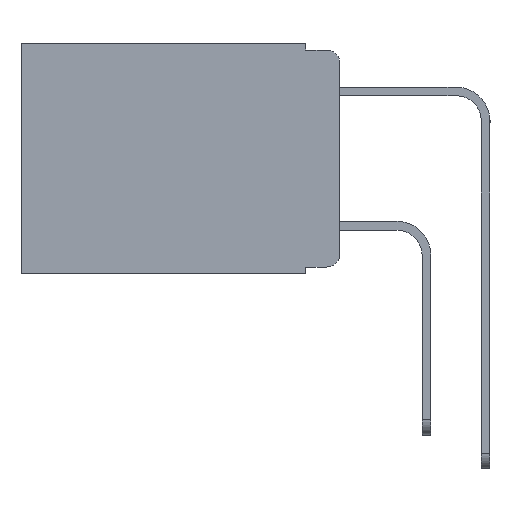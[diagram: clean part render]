
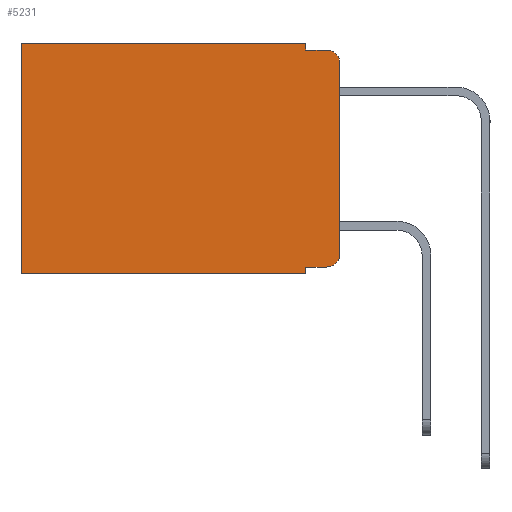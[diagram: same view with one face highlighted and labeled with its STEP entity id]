
A CAD part, left-side view. The second image highlights one B-rep face of the part: STEP entity #5231.
In plain terms, the highlighted planar face has unit normal (-1, 0, 0).
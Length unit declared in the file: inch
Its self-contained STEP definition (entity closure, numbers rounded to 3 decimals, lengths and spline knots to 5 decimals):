
#2 = CARTESIAN_POINT ( 'NONE',  ( 0.298, 0.051, -0.343 ) ) ;
#319 = VERTEX_POINT ( 'NONE', #9623 ) ;
#1503 = CARTESIAN_POINT ( 'NONE',  ( 0.298, 0., -0.343 ) ) ;
#2318 = VERTEX_POINT ( 'NONE', #15195 ) ;
#2337 = ORIENTED_EDGE ( 'NONE', *, *, #12186, .F. ) ;
#2432 = VERTEX_POINT ( 'NONE', #8522 ) ;
#2642 = CARTESIAN_POINT ( 'NONE',  ( 0.298, 0.051, -0.333 ) ) ;
#3061 = VECTOR ( 'NONE', #10099, 39.37008 ) ;
#3215 = CIRCLE ( 'NONE', #21609, 0.02 ) ;
#3262 = ORIENTED_EDGE ( 'NONE', *, *, #10508, .F. ) ;
#3624 = EDGE_CURVE ( 'NONE', #319, #16542, #11801, .T. ) ;
#3670 = DIRECTION ( 'NONE',  ( 1., 0., 0. ) ) ;
#3845 = EDGE_LOOP ( 'NONE', ( #17991, #7827, #21614, #2337, #16322, #11525, #3848, #3262, #21906, #20778 ) ) ;
#3848 = ORIENTED_EDGE ( 'NONE', *, *, #21230, .F. ) ;
#3927 = CARTESIAN_POINT ( 'NONE',  ( 0.298, 0.473, 0. ) ) ;
#3942 = EDGE_CURVE ( 'NONE', #23337, #8528, #10351, .T. ) ;
#4706 = VECTOR ( 'NONE', #10716, 39.37008 ) ;
#4889 = CARTESIAN_POINT ( 'NONE',  ( 0.298, 0.051, -0.01 ) ) ;
#5173 = EDGE_CURVE ( 'NONE', #8528, #9695, #3215, .T. ) ;
#5231 = ADVANCED_FACE ( 'NONE', ( #21304 ), #14564, .F. ) ;
#5513 = VECTOR ( 'NONE', #11139, 39.37008 ) ;
#5578 = DIRECTION ( 'NONE',  ( 0., -1., 0. ) ) ;
#5668 = VECTOR ( 'NONE', #12463, 39.37008 ) ;
#6241 = LINE ( 'NONE', #17768, #5668 ) ;
#6376 = VECTOR ( 'NONE', #5578, 39.37008 ) ;
#6674 = DIRECTION ( 'NONE',  ( 0., 0., -1. ) ) ;
#6680 = AXIS2_PLACEMENT_3D ( 'NONE', #23438, #3670, #16369 ) ;
#7228 = CARTESIAN_POINT ( 'NONE',  ( 0.298, 0.02, -0.01 ) ) ;
#7505 = VECTOR ( 'NONE', #14910, 39.37008 ) ;
#7630 = DIRECTION ( 'NONE',  ( 0., 0., -1. ) ) ;
#7827 = ORIENTED_EDGE ( 'NONE', *, *, #22779, .T. ) ;
#8060 = LINE ( 'NONE', #13087, #7505 ) ;
#8366 = EDGE_CURVE ( 'NONE', #15752, #9695, #8524, .T. ) ;
#8522 = CARTESIAN_POINT ( 'NONE',  ( 0.298, 0.051, 0. ) ) ;
#8524 = LINE ( 'NONE', #11943, #3061 ) ;
#8528 = VERTEX_POINT ( 'NONE', #17709 ) ;
#8738 = DIRECTION ( 'NONE',  ( -1., 0., 0. ) ) ;
#9536 = LINE ( 'NONE', #18415, #15468 ) ;
#9623 = CARTESIAN_POINT ( 'NONE',  ( 0.298, 0.051, -0.01 ) ) ;
#9695 = VERTEX_POINT ( 'NONE', #16052 ) ;
#10099 = DIRECTION ( 'NONE',  ( 0., 0., -1. ) ) ;
#10351 = LINE ( 'NONE', #2642, #5513 ) ;
#10508 = EDGE_CURVE ( 'NONE', #23337, #15420, #9536, .T. ) ;
#10716 = DIRECTION ( 'NONE',  ( 0., 1., 0. ) ) ;
#10855 = CARTESIAN_POINT ( 'NONE',  ( 0.298, 0.02, -0.313 ) ) ;
#10963 = EDGE_CURVE ( 'NONE', #11187, #2318, #6241, .T. ) ;
#11139 = DIRECTION ( 'NONE',  ( 0., -1., 0. ) ) ;
#11187 = VERTEX_POINT ( 'NONE', #3927 ) ;
#11525 = ORIENTED_EDGE ( 'NONE', *, *, #10963, .T. ) ;
#11801 = LINE ( 'NONE', #4889, #6376 ) ;
#11943 = CARTESIAN_POINT ( 'NONE',  ( 0.298, 0., 0. ) ) ;
#12186 = EDGE_CURVE ( 'NONE', #2432, #319, #22229, .T. ) ;
#12463 = DIRECTION ( 'NONE',  ( 0., 0., -1. ) ) ;
#12674 = DIRECTION ( 'NONE',  ( 0., 0., -1. ) ) ;
#13087 = CARTESIAN_POINT ( 'NONE',  ( 0.298, 0., 0. ) ) ;
#14564 = PLANE ( 'NONE',  #6680 ) ;
#14567 = AXIS2_PLACEMENT_3D ( 'NONE', #19501, #8738, #21286 ) ;
#14910 = DIRECTION ( 'NONE',  ( 0., 1., 0. ) ) ;
#15195 = CARTESIAN_POINT ( 'NONE',  ( 0.298, 0.473, -0.343 ) ) ;
#15420 = VERTEX_POINT ( 'NONE', #2 ) ;
#15468 = VECTOR ( 'NONE', #7630, 39.37008 ) ;
#15687 = CARTESIAN_POINT ( 'NONE',  ( 0.298, 0., -0.03 ) ) ;
#15752 = VERTEX_POINT ( 'NONE', #15687 ) ;
#16052 = CARTESIAN_POINT ( 'NONE',  ( 0.298, 0., -0.313 ) ) ;
#16322 = ORIENTED_EDGE ( 'NONE', *, *, #22444, .T. ) ;
#16369 = DIRECTION ( 'NONE',  ( 0., 0., -1. ) ) ;
#16542 = VERTEX_POINT ( 'NONE', #7228 ) ;
#17500 = CARTESIAN_POINT ( 'NONE',  ( 0.298, 0.051, 0. ) ) ;
#17709 = CARTESIAN_POINT ( 'NONE',  ( 0.298, 0.02, -0.333 ) ) ;
#17768 = CARTESIAN_POINT ( 'NONE',  ( 0.298, 0.473, 0. ) ) ;
#17991 = ORIENTED_EDGE ( 'NONE', *, *, #8366, .F. ) ;
#18415 = CARTESIAN_POINT ( 'NONE',  ( 0.298, 0.051, 0. ) ) ;
#19098 = LINE ( 'NONE', #1503, #4706 ) ;
#19308 = CARTESIAN_POINT ( 'NONE',  ( 0.298, 0.051, -0.333 ) ) ;
#19501 = CARTESIAN_POINT ( 'NONE',  ( 0.298, 0.02, -0.03 ) ) ;
#20778 = ORIENTED_EDGE ( 'NONE', *, *, #5173, .T. ) ;
#21230 = EDGE_CURVE ( 'NONE', #15420, #2318, #19098, .T. ) ;
#21286 = DIRECTION ( 'NONE',  ( 0., 0., -1. ) ) ;
#21304 = FACE_OUTER_BOUND ( 'NONE', #3845, .T. ) ;
#21609 = AXIS2_PLACEMENT_3D ( 'NONE', #10855, #23357, #12674 ) ;
#21614 = ORIENTED_EDGE ( 'NONE', *, *, #3624, .F. ) ;
#21906 = ORIENTED_EDGE ( 'NONE', *, *, #3942, .T. ) ;
#22229 = LINE ( 'NONE', #17500, #22775 ) ;
#22444 = EDGE_CURVE ( 'NONE', #2432, #11187, #8060, .T. ) ;
#22775 = VECTOR ( 'NONE', #6674, 39.37008 ) ;
#22779 = EDGE_CURVE ( 'NONE', #15752, #16542, #23469, .T. ) ;
#23337 = VERTEX_POINT ( 'NONE', #19308 ) ;
#23357 = DIRECTION ( 'NONE',  ( -1., 0., 0. ) ) ;
#23438 = CARTESIAN_POINT ( 'NONE',  ( 0.298, 0., 0. ) ) ;
#23469 = CIRCLE ( 'NONE', #14567, 0.02 ) ;
